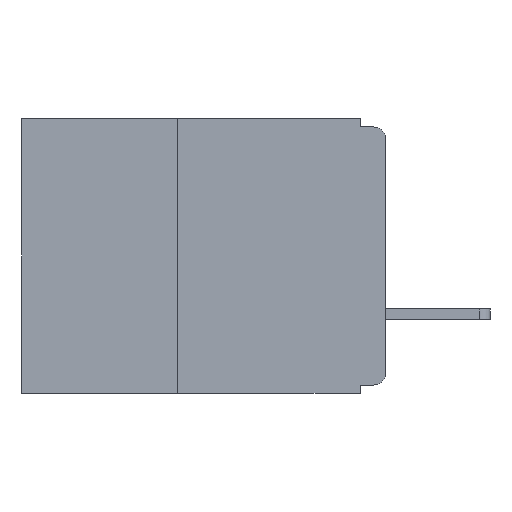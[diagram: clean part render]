
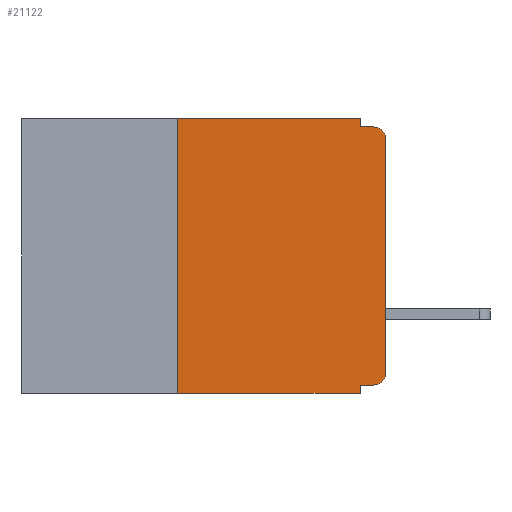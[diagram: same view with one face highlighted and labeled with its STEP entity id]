
A CAD part, left-side view. The second image highlights one B-rep face of the part: STEP entity #21122.
In plain terms, the highlighted planar face has unit normal (-1, 0, 0).
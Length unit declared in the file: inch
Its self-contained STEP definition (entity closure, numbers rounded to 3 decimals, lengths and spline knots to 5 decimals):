
#368 = VECTOR ( 'NONE', #11954, 39.37008 ) ;
#1528 = ORIENTED_EDGE ( 'NONE', *, *, #16655, .F. ) ;
#2607 = EDGE_CURVE ( 'NONE', #20036, #4811, #7514, .T. ) ;
#2690 = VECTOR ( 'NONE', #8496, 39.37008 ) ;
#3127 = PLANE ( 'NONE',  #6783 ) ;
#3262 = CARTESIAN_POINT ( 'NONE',  ( 0., 0.031, -0.32 ) ) ;
#3366 = ORIENTED_EDGE ( 'NONE', *, *, #12272, .T. ) ;
#4290 = DIRECTION ( 'NONE',  ( 0., 0., 1. ) ) ;
#4393 = CARTESIAN_POINT ( 'NONE',  ( 0., 0.25, -0.33 ) ) ;
#4811 = VERTEX_POINT ( 'NONE', #17061 ) ;
#5285 = ORIENTED_EDGE ( 'NONE', *, *, #21556, .F. ) ;
#5757 = VERTEX_POINT ( 'NONE', #12943 ) ;
#6099 = VERTEX_POINT ( 'NONE', #17215 ) ;
#6255 = VERTEX_POINT ( 'NONE', #12174 ) ;
#6441 = VECTOR ( 'NONE', #9174, 39.37008 ) ;
#6474 = ORIENTED_EDGE ( 'NONE', *, *, #14592, .T. ) ;
#6611 = DIRECTION ( 'NONE',  ( 0., -1., 0. ) ) ;
#6645 = CARTESIAN_POINT ( 'NONE',  ( 0., 0., -0.32 ) ) ;
#6783 = AXIS2_PLACEMENT_3D ( 'NONE', #19634, #8592, #21513 ) ;
#6852 = LINE ( 'NONE', #4393, #10584 ) ;
#6904 = LINE ( 'NONE', #6645, #2690 ) ;
#6952 = DIRECTION ( 'NONE',  ( -1., 0., 0. ) ) ;
#7265 = CARTESIAN_POINT ( 'NONE',  ( 0., 0.015, -0.305 ) ) ;
#7514 = CIRCLE ( 'NONE', #20659, 0.015 ) ;
#8019 = CARTESIAN_POINT ( 'NONE',  ( 0., 0.031, 0. ) ) ;
#8354 = VERTEX_POINT ( 'NONE', #16114 ) ;
#8496 = DIRECTION ( 'NONE',  ( 0., 1., 0. ) ) ;
#8592 = DIRECTION ( 'NONE',  ( 1., 0., 0. ) ) ;
#9053 = CARTESIAN_POINT ( 'NONE',  ( 0., 0.015, -0.32 ) ) ;
#9100 = CIRCLE ( 'NONE', #11568, 0.015 ) ;
#9174 = DIRECTION ( 'NONE',  ( 0., 0., 1. ) ) ;
#9465 = EDGE_CURVE ( 'NONE', #8354, #21818, #6852, .T. ) ;
#9507 = DIRECTION ( 'NONE',  ( 0., 0., -1. ) ) ;
#9538 = VERTEX_POINT ( 'NONE', #3262 ) ;
#10130 = LINE ( 'NONE', #19432, #19391 ) ;
#10172 = DIRECTION ( 'NONE',  ( -1., 0., 0. ) ) ;
#10335 = VECTOR ( 'NONE', #15595, 39.37008 ) ;
#10584 = VECTOR ( 'NONE', #4290, 39.37008 ) ;
#10801 = EDGE_CURVE ( 'NONE', #6255, #6099, #14298, .T. ) ;
#11337 = ORIENTED_EDGE ( 'NONE', *, *, #10801, .F. ) ;
#11568 = AXIS2_PLACEMENT_3D ( 'NONE', #21260, #10172, #23081 ) ;
#11954 = DIRECTION ( 'NONE',  ( 0., 0., -1. ) ) ;
#12174 = CARTESIAN_POINT ( 'NONE',  ( 0., 0.031, -0.01 ) ) ;
#12272 = EDGE_CURVE ( 'NONE', #4811, #5757, #21155, .T. ) ;
#12943 = CARTESIAN_POINT ( 'NONE',  ( 0., 0., -0.025 ) ) ;
#13158 = VERTEX_POINT ( 'NONE', #15009 ) ;
#13410 = EDGE_CURVE ( 'NONE', #21818, #13158, #10130, .T. ) ;
#13461 = VERTEX_POINT ( 'NONE', #15897 ) ;
#13606 = DIRECTION ( 'NONE',  ( 0., 0., -1. ) ) ;
#13752 = CARTESIAN_POINT ( 'NONE',  ( 0., 0.437, -0.33 ) ) ;
#14078 = DIRECTION ( 'NONE',  ( 0., -1., 0. ) ) ;
#14298 = LINE ( 'NONE', #17766, #19198 ) ;
#14592 = EDGE_CURVE ( 'NONE', #8354, #13461, #15864, .T. ) ;
#14801 = ORIENTED_EDGE ( 'NONE', *, *, #19801, .T. ) ;
#15009 = CARTESIAN_POINT ( 'NONE',  ( 0., 0.031, 0. ) ) ;
#15258 = VECTOR ( 'NONE', #13606, 39.37008 ) ;
#15427 = ORIENTED_EDGE ( 'NONE', *, *, #9465, .F. ) ;
#15595 = DIRECTION ( 'NONE',  ( 0., -1., 0. ) ) ;
#15864 = LINE ( 'NONE', #13752, #10335 ) ;
#15878 = FACE_OUTER_BOUND ( 'NONE', #23010, .T. ) ;
#15897 = CARTESIAN_POINT ( 'NONE',  ( 0., 0.031, -0.33 ) ) ;
#16114 = CARTESIAN_POINT ( 'NONE',  ( 0., 0.25, -0.33 ) ) ;
#16506 = CARTESIAN_POINT ( 'NONE',  ( 0., 0., 0. ) ) ;
#16655 = EDGE_CURVE ( 'NONE', #20036, #9538, #6904, .T. ) ;
#17061 = CARTESIAN_POINT ( 'NONE',  ( 0., 0., -0.305 ) ) ;
#17212 = EDGE_CURVE ( 'NONE', #9538, #13461, #18707, .T. ) ;
#17215 = CARTESIAN_POINT ( 'NONE',  ( 0., 0.015, -0.01 ) ) ;
#17308 = ORIENTED_EDGE ( 'NONE', *, *, #17212, .F. ) ;
#17766 = CARTESIAN_POINT ( 'NONE',  ( 0., 0., -0.01 ) ) ;
#18307 = CARTESIAN_POINT ( 'NONE',  ( 0., 0.25, 0. ) ) ;
#18707 = LINE ( 'NONE', #22970, #368 ) ;
#19198 = VECTOR ( 'NONE', #14078, 39.37008 ) ;
#19391 = VECTOR ( 'NONE', #6611, 39.37008 ) ;
#19432 = CARTESIAN_POINT ( 'NONE',  ( 0., 0.437, 0. ) ) ;
#19634 = CARTESIAN_POINT ( 'NONE',  ( 0., 0.437, 0. ) ) ;
#19647 = ORIENTED_EDGE ( 'NONE', *, *, #13410, .F. ) ;
#19801 = EDGE_CURVE ( 'NONE', #5757, #6099, #9100, .T. ) ;
#20036 = VERTEX_POINT ( 'NONE', #9053 ) ;
#20157 = LINE ( 'NONE', #8019, #15258 ) ;
#20659 = AXIS2_PLACEMENT_3D ( 'NONE', #7265, #6952, #9507 ) ;
#21122 = ADVANCED_FACE ( 'NONE', ( #15878 ), #3127, .F. ) ;
#21155 = LINE ( 'NONE', #16506, #6441 ) ;
#21260 = CARTESIAN_POINT ( 'NONE',  ( 0., 0.015, -0.025 ) ) ;
#21513 = DIRECTION ( 'NONE',  ( 0., 0., -1. ) ) ;
#21556 = EDGE_CURVE ( 'NONE', #13158, #6255, #20157, .T. ) ;
#21632 = ORIENTED_EDGE ( 'NONE', *, *, #2607, .T. ) ;
#21818 = VERTEX_POINT ( 'NONE', #18307 ) ;
#22970 = CARTESIAN_POINT ( 'NONE',  ( 0., 0.031, -0.33 ) ) ;
#23010 = EDGE_LOOP ( 'NONE', ( #3366, #14801, #11337, #5285, #19647, #15427, #6474, #17308, #1528, #21632 ) ) ;
#23081 = DIRECTION ( 'NONE',  ( 0., 0., -1. ) ) ;
